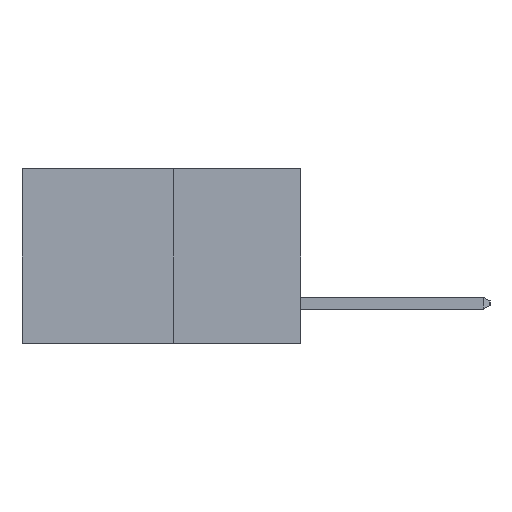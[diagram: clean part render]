
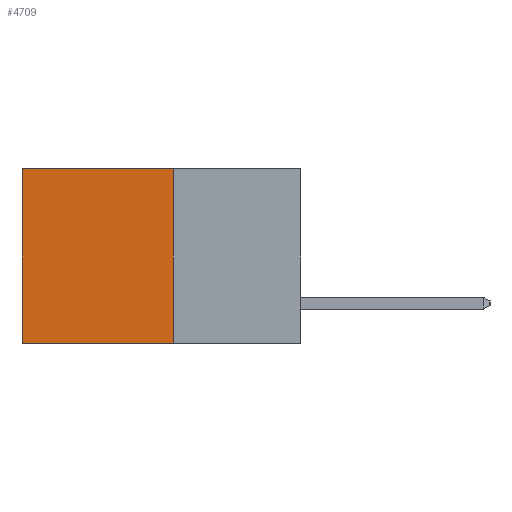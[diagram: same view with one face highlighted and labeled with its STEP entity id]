
A CAD part, left-side view. The second image highlights one B-rep face of the part: STEP entity #4709.
In plain terms, the highlighted planar face has unit normal (-1, 0, 0).
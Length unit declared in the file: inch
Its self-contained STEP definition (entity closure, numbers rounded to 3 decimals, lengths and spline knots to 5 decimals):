
#486 = CARTESIAN_POINT ( 'NONE',  ( 0.277, 0.27, 0. ) ) ;
#1239 = CARTESIAN_POINT ( 'NONE',  ( 0.277, 0.27, -0.37 ) ) ;
#1259 = DIRECTION ( 'NONE',  ( 0., 1., 0. ) ) ;
#1653 = CARTESIAN_POINT ( 'NONE',  ( 0.277, 0.27, -0.37 ) ) ;
#2165 = DIRECTION ( 'NONE',  ( 1., 0., 0. ) ) ;
#2503 = PLANE ( 'NONE',  #9890 ) ;
#2556 = ORIENTED_EDGE ( 'NONE', *, *, #7689, .T. ) ;
#2567 = ORIENTED_EDGE ( 'NONE', *, *, #8645, .F. ) ;
#2599 = ORIENTED_EDGE ( 'NONE', *, *, #9383, .F. ) ;
#2608 = ORIENTED_EDGE ( 'NONE', *, *, #13416, .T. ) ;
#2611 = VECTOR ( 'NONE', #8059, 39.37008 ) ;
#2708 = LINE ( 'NONE', #2728, #13349 ) ;
#2728 = CARTESIAN_POINT ( 'NONE',  ( 0.277, 0.27, -0.37 ) ) ;
#4709 = ADVANCED_FACE ( 'NONE', ( #11984 ), #2503, .F. ) ;
#4868 = CARTESIAN_POINT ( 'NONE',  ( 0.277, 0.27, 0. ) ) ;
#6475 = LINE ( 'NONE', #1239, #11599 ) ;
#6784 = EDGE_LOOP ( 'NONE', ( #2556, #2567, #2599, #2608 ) ) ;
#7689 = EDGE_CURVE ( 'NONE', #7780, #11189, #10939, .T. ) ;
#7780 = VERTEX_POINT ( 'NONE', #9558 ) ;
#7847 = VERTEX_POINT ( 'NONE', #9115 ) ;
#7881 = DIRECTION ( 'NONE',  ( 0., 0., -1. ) ) ;
#8059 = DIRECTION ( 'NONE',  ( 0., 1., 0. ) ) ;
#8573 = VECTOR ( 'NONE', #10344, 39.37008 ) ;
#8645 = EDGE_CURVE ( 'NONE', #7847, #11189, #6475, .T. ) ;
#9115 = CARTESIAN_POINT ( 'NONE',  ( 0.277, 0.27, -0.37 ) ) ;
#9383 = EDGE_CURVE ( 'NONE', #12653, #7847, #2708, .T. ) ;
#9558 = CARTESIAN_POINT ( 'NONE',  ( 0.277, 0.59, 0. ) ) ;
#9890 = AXIS2_PLACEMENT_3D ( 'NONE', #1653, #2165, #7881 ) ;
#10344 = DIRECTION ( 'NONE',  ( 0., 0., -1. ) ) ;
#10376 = CARTESIAN_POINT ( 'NONE',  ( 0.277, 0.59, -0.37 ) ) ;
#10939 = LINE ( 'NONE', #10376, #8573 ) ;
#11003 = LINE ( 'NONE', #486, #2611 ) ;
#11153 = DIRECTION ( 'NONE',  ( 0., 0., -1. ) ) ;
#11189 = VERTEX_POINT ( 'NONE', #12905 ) ;
#11599 = VECTOR ( 'NONE', #1259, 39.37008 ) ;
#11984 = FACE_OUTER_BOUND ( 'NONE', #6784, .T. ) ;
#12653 = VERTEX_POINT ( 'NONE', #4868 ) ;
#12905 = CARTESIAN_POINT ( 'NONE',  ( 0.277, 0.59, -0.37 ) ) ;
#13349 = VECTOR ( 'NONE', #11153, 39.37008 ) ;
#13416 = EDGE_CURVE ( 'NONE', #12653, #7780, #11003, .T. ) ;
